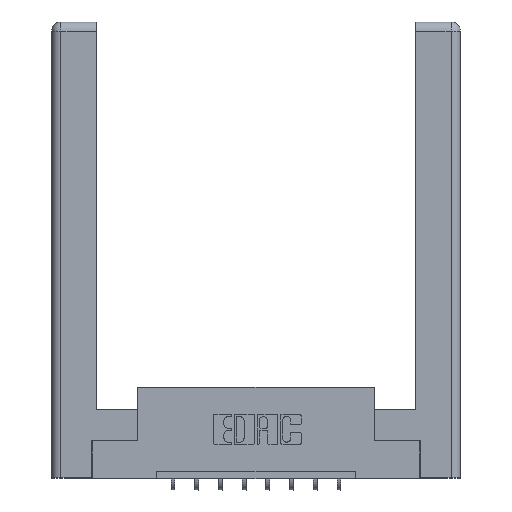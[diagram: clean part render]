
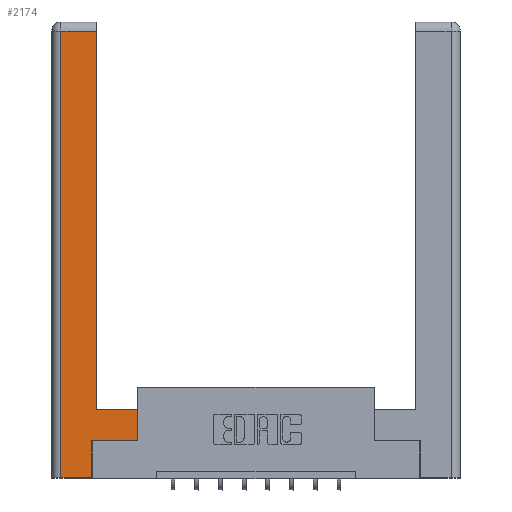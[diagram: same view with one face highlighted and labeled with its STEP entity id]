
A CAD part, top view. The second image highlights one B-rep face of the part: STEP entity #2174.
In plain terms, the highlighted planar face has unit normal (0, 0, 1).
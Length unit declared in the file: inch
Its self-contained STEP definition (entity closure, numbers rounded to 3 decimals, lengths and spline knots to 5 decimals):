
#73 = DIRECTION ( 'NONE',  ( 0., 1., 0. ) ) ;
#96 = VERTEX_POINT ( 'NONE', #12825 ) ;
#200 = CARTESIAN_POINT ( 'NONE',  ( 0.265, 0.245, 0. ) ) ;
#335 = EDGE_CURVE ( 'NONE', #10563, #6458, #10438, .T. ) ;
#407 = CARTESIAN_POINT ( 'NONE',  ( 0.295, 3., 0. ) ) ;
#463 = DIRECTION ( 'NONE',  ( -1., 0., 0. ) ) ;
#739 = EDGE_CURVE ( 'NONE', #11918, #10563, #11290, .T. ) ;
#790 = DIRECTION ( 'NONE',  ( 0., -1., 0. ) ) ;
#958 = VECTOR ( 'NONE', #11379, 39.37008 ) ;
#1163 = AXIS2_PLACEMENT_3D ( 'NONE', #7709, #4680, #463 ) ;
#1171 = VECTOR ( 'NONE', #5309, 39.37008 ) ;
#1232 = LINE ( 'NONE', #2094, #8411 ) ;
#1866 = EDGE_CURVE ( 'NONE', #12686, #4467, #2378, .T. ) ;
#2094 = CARTESIAN_POINT ( 'NONE',  ( 0.565, 0.245, 0. ) ) ;
#2174 = ADVANCED_FACE ( 'NONE', ( #6106 ), #2557, .F. ) ;
#2378 = LINE ( 'NONE', #200, #5132 ) ;
#2406 = DIRECTION ( 'NONE',  ( 0., 1., 0. ) ) ;
#2445 = ORIENTED_EDGE ( 'NONE', *, *, #10890, .T. ) ;
#2557 = PLANE ( 'NONE',  #1163 ) ;
#2850 = CARTESIAN_POINT ( 'NONE',  ( 0.565, 0.245, 0. ) ) ;
#3390 = VECTOR ( 'NONE', #4974, 39.37008 ) ;
#3439 = EDGE_CURVE ( 'NONE', #6458, #6705, #12954, .T. ) ;
#3990 = CARTESIAN_POINT ( 'NONE',  ( 0.265, 0., 0. ) ) ;
#4467 = VERTEX_POINT ( 'NONE', #9664 ) ;
#4523 = EDGE_CURVE ( 'NONE', #4467, #11918, #1232, .T. ) ;
#4535 = ORIENTED_EDGE ( 'NONE', *, *, #3439, .T. ) ;
#4680 = DIRECTION ( 'NONE',  ( 0., 0., -1. ) ) ;
#4974 = DIRECTION ( 'NONE',  ( 1., 0., 0. ) ) ;
#5044 = EDGE_LOOP ( 'NONE', ( #4535, #5509, #5951, #2445, #11437, #9831, #11653, #10489 ) ) ;
#5132 = VECTOR ( 'NONE', #73, 39.37008 ) ;
#5309 = DIRECTION ( 'NONE',  ( 0., 1., 0. ) ) ;
#5444 = VECTOR ( 'NONE', #2406, 39.37008 ) ;
#5509 = ORIENTED_EDGE ( 'NONE', *, *, #7729, .T. ) ;
#5951 = ORIENTED_EDGE ( 'NONE', *, *, #13049, .T. ) ;
#6106 = FACE_OUTER_BOUND ( 'NONE', #5044, .T. ) ;
#6359 = CARTESIAN_POINT ( 'NONE',  ( 0.0615, 2.94, 0. ) ) ;
#6458 = VERTEX_POINT ( 'NONE', #12772 ) ;
#6469 = LINE ( 'NONE', #3990, #3390 ) ;
#6559 = CARTESIAN_POINT ( 'NONE',  ( 0.265, 0., 0. ) ) ;
#6705 = VERTEX_POINT ( 'NONE', #8728 ) ;
#6833 = CARTESIAN_POINT ( 'NONE',  ( 0.0615, 0., 0. ) ) ;
#7498 = DIRECTION ( 'NONE',  ( -1., 0., 0. ) ) ;
#7709 = CARTESIAN_POINT ( 'NONE',  ( 0., 0., 0. ) ) ;
#7729 = EDGE_CURVE ( 'NONE', #6705, #12202, #11297, .T. ) ;
#8264 = CARTESIAN_POINT ( 'NONE',  ( 0.295, 0.45, 0. ) ) ;
#8411 = VECTOR ( 'NONE', #11217, 39.37008 ) ;
#8728 = CARTESIAN_POINT ( 'NONE',  ( 0.295, 2.94, 0. ) ) ;
#9019 = LINE ( 'NONE', #6833, #11955 ) ;
#9664 = CARTESIAN_POINT ( 'NONE',  ( 0.265, 0.245, 0. ) ) ;
#9831 = ORIENTED_EDGE ( 'NONE', *, *, #4523, .T. ) ;
#9865 = CARTESIAN_POINT ( 'NONE',  ( 0.0615, 2.94, 0. ) ) ;
#10222 = VECTOR ( 'NONE', #7498, 39.37008 ) ;
#10438 = LINE ( 'NONE', #8264, #958 ) ;
#10489 = ORIENTED_EDGE ( 'NONE', *, *, #335, .T. ) ;
#10563 = VERTEX_POINT ( 'NONE', #12407 ) ;
#10890 = EDGE_CURVE ( 'NONE', #96, #12686, #6469, .T. ) ;
#11217 = DIRECTION ( 'NONE',  ( 1., 0., 0. ) ) ;
#11290 = LINE ( 'NONE', #12447, #1171 ) ;
#11297 = LINE ( 'NONE', #6359, #10222 ) ;
#11379 = DIRECTION ( 'NONE',  ( -1., 0., 0. ) ) ;
#11437 = ORIENTED_EDGE ( 'NONE', *, *, #1866, .T. ) ;
#11653 = ORIENTED_EDGE ( 'NONE', *, *, #739, .T. ) ;
#11918 = VERTEX_POINT ( 'NONE', #2850 ) ;
#11955 = VECTOR ( 'NONE', #790, 39.37008 ) ;
#12202 = VERTEX_POINT ( 'NONE', #9865 ) ;
#12407 = CARTESIAN_POINT ( 'NONE',  ( 0.565, 0.45, 0. ) ) ;
#12447 = CARTESIAN_POINT ( 'NONE',  ( 0.565, 0.45, 0. ) ) ;
#12686 = VERTEX_POINT ( 'NONE', #6559 ) ;
#12772 = CARTESIAN_POINT ( 'NONE',  ( 0.295, 0.45, 0. ) ) ;
#12825 = CARTESIAN_POINT ( 'NONE',  ( 0.0615, 0., 0. ) ) ;
#12954 = LINE ( 'NONE', #407, #5444 ) ;
#13049 = EDGE_CURVE ( 'NONE', #12202, #96, #9019, .T. ) ;
